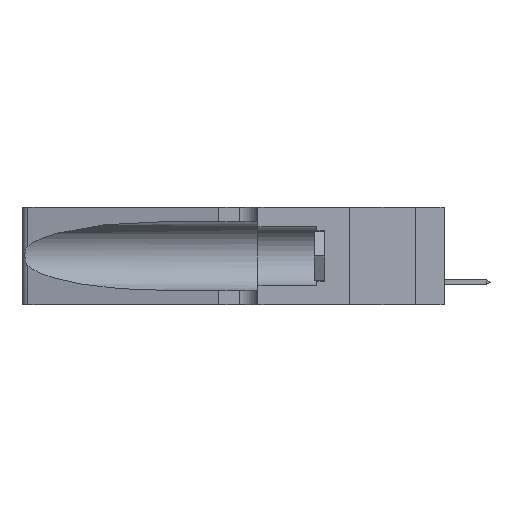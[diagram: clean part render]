
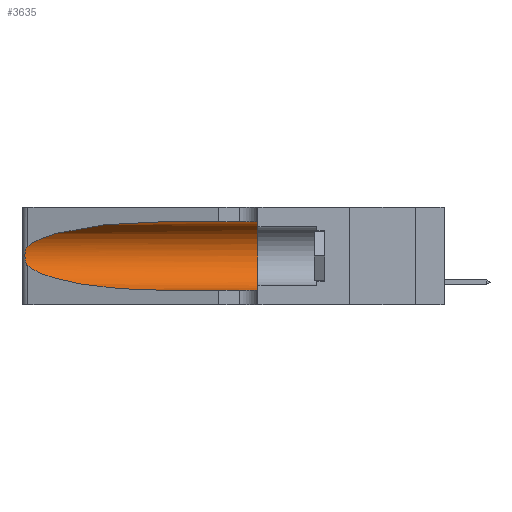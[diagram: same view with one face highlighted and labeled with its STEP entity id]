
A CAD part, left-side view. The second image highlights one B-rep face of the part: STEP entity #3635.
In plain terms, the highlighted cylindrical face has radius 3.308 mm (diameter 6.617 mm), a partial arc.
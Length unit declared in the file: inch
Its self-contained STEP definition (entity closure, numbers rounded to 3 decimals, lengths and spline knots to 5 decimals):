
#463 = CARTESIAN_POINT ( 'NONE',  ( 0.25639, 1.23184, 0.21858 ) ) ;
#739 = CARTESIAN_POINT ( 'NONE',  ( 0.26017, 1.23833, 0.17102 ) ) ;
#801 = VERTEX_POINT ( 'NONE', #13485 ) ;
#1922 =( BOUNDED_CURVE ( )  B_SPLINE_CURVE ( 3, ( #25395, #2868, #21959, #35051 ),
 .UNSPECIFIED., .F., .F. ) 
 B_SPLINE_CURVE_WITH_KNOTS ( ( 4, 4 ),
 ( 3.44316, 4.71239 ),
 .UNSPECIFIED. ) 
 CURVE ( )  GEOMETRIC_REPRESENTATION_ITEM ( )  RATIONAL_B_SPLINE_CURVE ( ( 1., 0.87, 0.87, 1. ) ) 
 REPRESENTATION_ITEM ( '' )  );
#2076 = CARTESIAN_POINT ( 'NONE',  ( 0.25487, 1.22718, 0.22369 ) ) ;
#2868 = CARTESIAN_POINT ( 'NONE',  ( 0.2373, 1.15595, 0.08982 ) ) ;
#2909 = VERTEX_POINT ( 'NONE', #20410 ) ;
#3635 = ADVANCED_FACE ( 'NONE', ( #13078 ), #19154, .F. ) ;
#3745 = CARTESIAN_POINT ( 'NONE',  ( 0.25787, 1.23484, 0.2124 ) ) ;
#3850 = VERTEX_POINT ( 'NONE', #2076 ) ;
#4173 = CARTESIAN_POINT ( 'NONE',  ( 0.25856, 1.23593, 0.16098 ) ) ;
#5008 = CARTESIAN_POINT ( 'NONE',  ( 0.1305, 1.61858, 0.05475 ) ) ;
#6112 = ORIENTED_EDGE ( 'NONE', *, *, #29544, .T. ) ;
#7150 = CARTESIAN_POINT ( 'NONE',  ( 0.25854, 1.2359, 0.20912 ) ) ;
#7796 = CIRCLE ( 'NONE', #20983, 0.13025 ) ;
#9576 = VERTEX_POINT ( 'NONE', #15130 ) ;
#10243 = CARTESIAN_POINT ( 'NONE',  ( 0.26018, 1.23835, 0.19895 ) ) ;
#10533 = ORIENTED_EDGE ( 'NONE', *, *, #23086, .F. ) ;
#11394 = CARTESIAN_POINT ( 'NONE',  ( 0.25487, 1.22718, 0.22369 ) ) ;
#12938 = DIRECTION ( 'NONE',  ( 0., -1., 0. ) ) ;
#13078 = FACE_OUTER_BOUND ( 'NONE', #16294, .T. ) ;
#13485 = CARTESIAN_POINT ( 'NONE',  ( 0.1305, 0.72297, 0.31525 ) ) ;
#13652 = CARTESIAN_POINT ( 'NONE',  ( 0.26075, 1.23896, 0.19203 ) ) ;
#15130 = CARTESIAN_POINT ( 'NONE',  ( 0.1305, 0.72297, 0.05475 ) ) ;
#16294 = EDGE_LOOP ( 'NONE', ( #35463, #19101, #32741, #6112, #35044, #10533 ) ) ;
#16412 = CARTESIAN_POINT ( 'NONE',  ( 0.1305, 0.35, 0.31525 ) ) ;
#16587 = VECTOR ( 'NONE', #12938, 39.37008 ) ;
#18129 = CARTESIAN_POINT ( 'NONE',  ( 0.1305, 0.35, 0.05475 ) ) ;
#18891 = CARTESIAN_POINT ( 'NONE',  ( 0.1305, 1.61858, 0.31525 ) ) ;
#19101 = ORIENTED_EDGE ( 'NONE', *, *, #19613, .T. ) ;
#19154 = CYLINDRICAL_SURFACE ( 'NONE', #40461, 0.13025 ) ;
#19613 = EDGE_CURVE ( 'NONE', #3850, #2909, #41723, .T. ) ;
#20410 = CARTESIAN_POINT ( 'NONE',  ( 0.25487, 1.22718, 0.14631 ) ) ;
#20449 = CARTESIAN_POINT ( 'NONE',  ( 0.25487, 1.22718, 0.22369 ) ) ;
#20983 = AXIS2_PLACEMENT_3D ( 'NONE', #32659, #34103, #33664 ) ;
#21266 = DIRECTION ( 'NONE',  ( 0., -1., 0. ) ) ;
#21959 = CARTESIAN_POINT ( 'NONE',  ( 0.18966, 0.96281, 0.05475 ) ) ;
#22692 = LINE ( 'NONE', #18891, #16587 ) ;
#23086 = EDGE_CURVE ( 'NONE', #801, #26496, #22692, .T. ) ;
#23153 = CARTESIAN_POINT ( 'NONE',  ( 0.25555, 1.22993, 0.14849 ) ) ;
#23708 = DIRECTION ( 'NONE',  ( 0., 0., -1. ) ) ;
#24279 = DIRECTION ( 'NONE',  ( 0., -1., 0. ) ) ;
#24720 = CARTESIAN_POINT ( 'NONE',  ( 0.2373, 1.15595, 0.28018 ) ) ;
#24756 = EDGE_CURVE ( 'NONE', #26496, #26121, #7796, .T. ) ;
#25395 = CARTESIAN_POINT ( 'NONE',  ( 0.25487, 1.22718, 0.14631 ) ) ;
#26121 = VERTEX_POINT ( 'NONE', #18129 ) ;
#26431 = CARTESIAN_POINT ( 'NONE',  ( 0.25789, 1.23486, 0.15765 ) ) ;
#26496 = VERTEX_POINT ( 'NONE', #16412 ) ;
#26721 = CARTESIAN_POINT ( 'NONE',  ( 0.26075, 1.23896, 0.178 ) ) ;
#27505 = VECTOR ( 'NONE', #21266, 39.37008 ) ;
#27734 = EDGE_CURVE ( 'NONE', #2909, #9576, #1922, .T. ) ;
#27908 =( BOUNDED_CURVE ( )  B_SPLINE_CURVE ( 3, ( #32976, #29850, #24720, #11394 ),
 .UNSPECIFIED., .F., .F. ) 
 B_SPLINE_CURVE_WITH_KNOTS ( ( 4, 4 ),
 ( 1.5708, 2.84003 ),
 .UNSPECIFIED. ) 
 CURVE ( )  GEOMETRIC_REPRESENTATION_ITEM ( )  RATIONAL_B_SPLINE_CURVE ( ( 1., 0.87, 0.87, 1. ) ) 
 REPRESENTATION_ITEM ( '' )  );
#29544 = EDGE_CURVE ( 'NONE', #9576, #26121, #41749, .T. ) ;
#29850 = CARTESIAN_POINT ( 'NONE',  ( 0.18966, 0.96281, 0.31525 ) ) ;
#29856 = CARTESIAN_POINT ( 'NONE',  ( 0.25555, 1.22994, 0.2215 ) ) ;
#29984 = CARTESIAN_POINT ( 'NONE',  ( 0.25639, 1.23186, 0.15144 ) ) ;
#32659 = CARTESIAN_POINT ( 'NONE',  ( 0.1305, 0.35, 0.185 ) ) ;
#32741 = ORIENTED_EDGE ( 'NONE', *, *, #27734, .T. ) ;
#32976 = CARTESIAN_POINT ( 'NONE',  ( 0.1305, 0.72297, 0.31525 ) ) ;
#33664 = DIRECTION ( 'NONE',  ( 0., 0., 1. ) ) ;
#33955 = CARTESIAN_POINT ( 'NONE',  ( 0.1305, 1.61858, 0.185 ) ) ;
#34103 = DIRECTION ( 'NONE',  ( 0., 1., 0. ) ) ;
#35044 = ORIENTED_EDGE ( 'NONE', *, *, #24756, .F. ) ;
#35051 = CARTESIAN_POINT ( 'NONE',  ( 0.1305, 0.72297, 0.05475 ) ) ;
#35463 = ORIENTED_EDGE ( 'NONE', *, *, #40877, .T. ) ;
#36638 = CARTESIAN_POINT ( 'NONE',  ( 0.25487, 1.22718, 0.14631 ) ) ;
#40461 = AXIS2_PLACEMENT_3D ( 'NONE', #33955, #24279, #23708 ) ;
#40877 = EDGE_CURVE ( 'NONE', #801, #3850, #27908, .T. ) ;
#41723 = B_SPLINE_CURVE_WITH_KNOTS ( 'NONE', 3,
 ( #20449, #29856, #463, #3745, #7150, #10243, #13652, #26721, #739, #4173, #26431, #29984, #23153, #36638 ),
 .UNSPECIFIED., .F., .F.,
 ( 4, 2, 2, 2, 2, 2, 4 ),
 ( 0., 0.00027, 0.00053, 0.00107, 0.0016, 0.00187, 0.00214 ),
 .UNSPECIFIED. ) ;
#41749 = LINE ( 'NONE', #5008, #27505 ) ;
